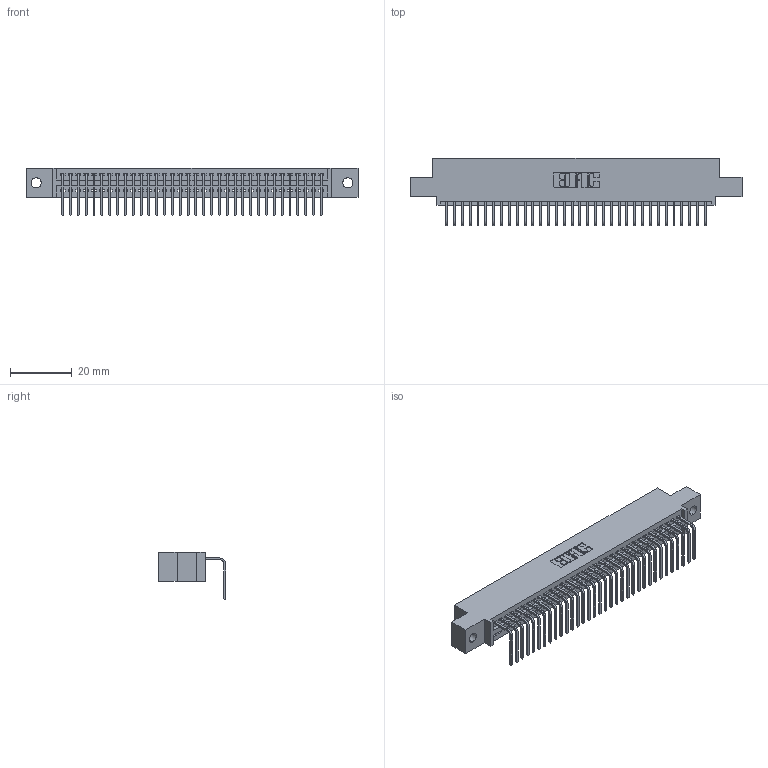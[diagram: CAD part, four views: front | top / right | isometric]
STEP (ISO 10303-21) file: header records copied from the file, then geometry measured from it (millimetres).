
FILE_DESCRIPTION (( 'STEP AP203' ), '1' );
FILE_NAME ('395-034-558-402.STEP', '2018-11-13T10:04:58', ( '' ), ( '' ), 'SwSTEP 2.0', 'SolidWorks 2016', '' );
FILE_SCHEMA (( 'CONFIG_CONTROL_DESIGN' ));
Length unit declared in the file: inch
Products named in the file (3): 345-292-001_558 Tail - 2; 395-034-558-402; 345 Part_0.110 Offset - 0.128 Dia
Assembly tree (35 placements, depth 2):
  395-034-558-402
    345 Part_0.110 Offset - 0.128 Dia
    345-292-001_558 Tail - 2  x34
Bounding box: 107.57 x 21.83 x 15.37 mm (x, y, z)
Volume: 10154.7 mm3; surface area: 13862 mm2
Topology: 35 solids, 35 shells, 2170 faces, 6541 edges, 4314 vertices
Faces by surface type: plane 1512, cylinder 658
Entity records: 26885 total; most frequent: CARTESIAN_POINT 4666, ORIENTED_EDGE 4634, DIRECTION 4085, EDGE_CURVE 2317, VECTOR 2049, LINE 2049, VERTEX_POINT 1542, AXIS2_PLACEMENT_3D 1018
